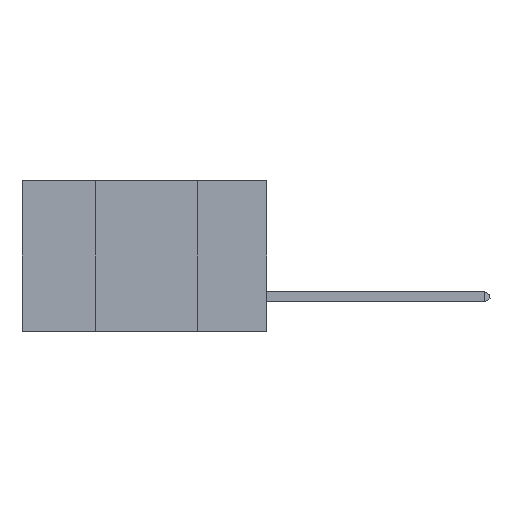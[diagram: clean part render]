
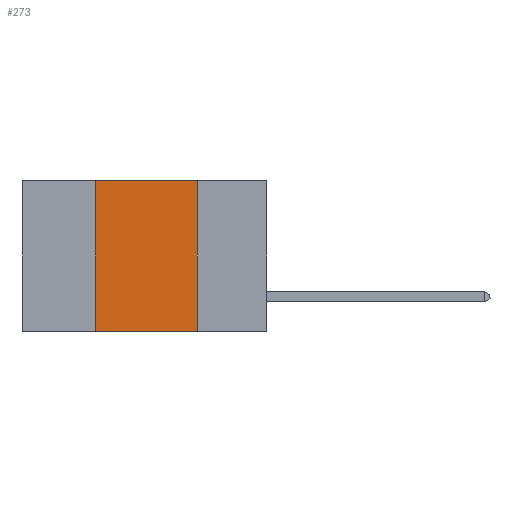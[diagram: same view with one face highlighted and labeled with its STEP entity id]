
A CAD part, left-side view. The second image highlights one B-rep face of the part: STEP entity #273.
In plain terms, the highlighted planar face has unit normal (-1, 0, 0).
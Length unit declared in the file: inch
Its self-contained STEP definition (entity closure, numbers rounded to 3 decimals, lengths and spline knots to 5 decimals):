
#273 = ADVANCED_FACE ( 'NONE', ( #8446 ), #11977, .F. ) ;
#1265 = DIRECTION ( 'NONE',  ( 0., 0., -1. ) ) ;
#1522 = DIRECTION ( 'NONE',  ( 0., 0., 1. ) ) ;
#2164 = EDGE_CURVE ( 'NONE', #8878, #19473, #16989, .T. ) ;
#2931 = CARTESIAN_POINT ( 'NONE',  ( 0., 0.17, 0. ) ) ;
#3499 = VECTOR ( 'NONE', #18262, 39.37008 ) ;
#3573 = DIRECTION ( 'NONE',  ( 0., -1., 0. ) ) ;
#4824 = LINE ( 'NONE', #11721, #9363 ) ;
#6257 = ORIENTED_EDGE ( 'NONE', *, *, #2164, .T. ) ;
#8446 = FACE_OUTER_BOUND ( 'NONE', #9721, .T. ) ;
#8878 = VERTEX_POINT ( 'NONE', #18477 ) ;
#9152 = LINE ( 'NONE', #2931, #21879 ) ;
#9327 = ORIENTED_EDGE ( 'NONE', *, *, #12462, .F. ) ;
#9363 = VECTOR ( 'NONE', #1522, 39.37008 ) ;
#9500 = VERTEX_POINT ( 'NONE', #11705 ) ;
#9721 = EDGE_LOOP ( 'NONE', ( #20195, #20228, #9327, #6257 ) ) ;
#10408 = CARTESIAN_POINT ( 'NONE',  ( 0., 0.6, 0. ) ) ;
#11705 = CARTESIAN_POINT ( 'NONE',  ( 0., 0.17, 0. ) ) ;
#11721 = CARTESIAN_POINT ( 'NONE',  ( 0., 0.42, 0. ) ) ;
#11977 = PLANE ( 'NONE',  #12904 ) ;
#12462 = EDGE_CURVE ( 'NONE', #8878, #19204, #4824, .T. ) ;
#12686 = DIRECTION ( 'NONE',  ( 1., 0., 0. ) ) ;
#12700 = DIRECTION ( 'NONE',  ( 0., 0., -1. ) ) ;
#12795 = LINE ( 'NONE', #10408, #16686 ) ;
#12904 = AXIS2_PLACEMENT_3D ( 'NONE', #14048, #12686, #12700 ) ;
#14048 = CARTESIAN_POINT ( 'NONE',  ( 0., 0.6, 0. ) ) ;
#16686 = VECTOR ( 'NONE', #3573, 39.37008 ) ;
#16972 = CARTESIAN_POINT ( 'NONE',  ( 0., 0.42, 0. ) ) ;
#16989 = LINE ( 'NONE', #18310, #3499 ) ;
#17203 = EDGE_CURVE ( 'NONE', #9500, #19473, #9152, .T. ) ;
#18262 = DIRECTION ( 'NONE',  ( 0., -1., 0. ) ) ;
#18310 = CARTESIAN_POINT ( 'NONE',  ( 0., 0.6, -0.37 ) ) ;
#18477 = CARTESIAN_POINT ( 'NONE',  ( 0., 0.42, -0.37 ) ) ;
#19204 = VERTEX_POINT ( 'NONE', #16972 ) ;
#19473 = VERTEX_POINT ( 'NONE', #20141 ) ;
#19572 = EDGE_CURVE ( 'NONE', #19204, #9500, #12795, .T. ) ;
#20141 = CARTESIAN_POINT ( 'NONE',  ( 0., 0.17, -0.37 ) ) ;
#20195 = ORIENTED_EDGE ( 'NONE', *, *, #17203, .F. ) ;
#20228 = ORIENTED_EDGE ( 'NONE', *, *, #19572, .F. ) ;
#21879 = VECTOR ( 'NONE', #1265, 39.37008 ) ;
